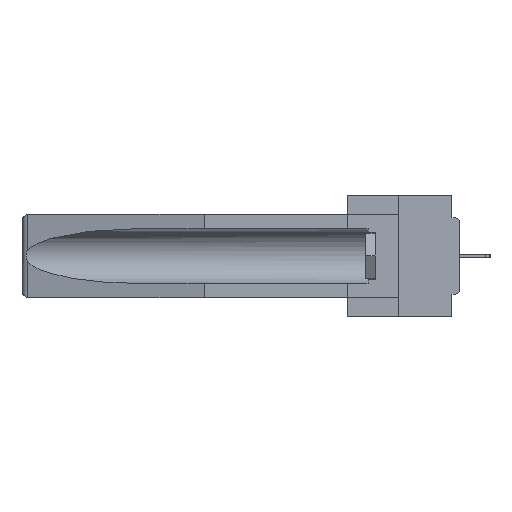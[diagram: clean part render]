
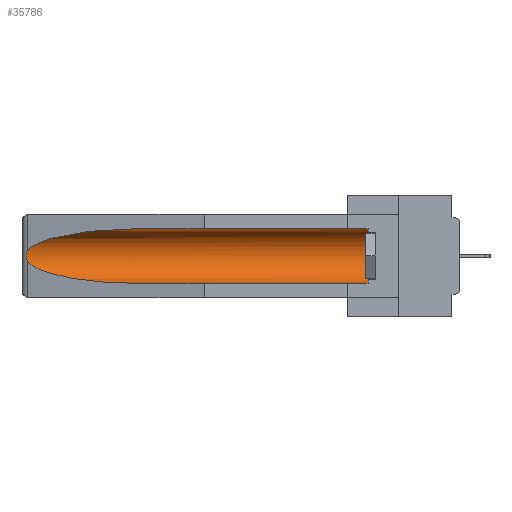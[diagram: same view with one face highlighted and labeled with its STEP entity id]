
A CAD part, left-side view. The second image highlights one B-rep face of the part: STEP entity #35786.
In plain terms, the highlighted cylindrical face has radius 2.857 mm (diameter 5.715 mm), a partial arc.
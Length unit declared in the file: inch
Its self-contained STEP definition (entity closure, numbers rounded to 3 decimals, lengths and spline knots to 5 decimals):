
#1238 = ORIENTED_EDGE ( 'NONE', *, *, #17198, .T. ) ;
#1365 = CARTESIAN_POINT ( 'NONE',  ( 0.2675, 1.53308, -0.16763 ) ) ;
#1535 = CYLINDRICAL_SURFACE ( 'NONE', #30972, 0.1125 ) ;
#1634 = VERTEX_POINT ( 'NONE', #39912 ) ;
#2962 = VERTEX_POINT ( 'NONE', #6089 ) ;
#3725 = CARTESIAN_POINT ( 'NONE',  ( 0.25451, 1.48313, -0.09465 ) ) ;
#5083 = CARTESIAN_POINT ( 'NONE',  ( 0.25451, 1.48313, -0.24835 ) ) ;
#6089 = CARTESIAN_POINT ( 'NONE',  ( 0.26537, 1.52718, -0.14972 ) ) ;
#6209 = ORIENTED_EDGE ( 'NONE', *, *, #26342, .T. ) ;
#6942 = CARTESIAN_POINT ( 'NONE',  ( 0.26654, 1.53092, -0.15636 ) ) ;
#7159 = EDGE_CURVE ( 'NONE', #2962, #30485, #22991, .T. ) ;
#7754 = CARTESIAN_POINT ( 'NONE',  ( 0.2673, 1.5327, -0.16383 ) ) ;
#8369 = CARTESIAN_POINT ( 'NONE',  ( 0.26537, 1.52718, -0.19328 ) ) ;
#9298 = DIRECTION ( 'NONE',  ( 0., 1., 0. ) ) ;
#13193 = CIRCLE ( 'NONE', #38894, 0.1125 ) ;
#13737 = CARTESIAN_POINT ( 'NONE',  ( 0.26537, 1.52718, -0.19328 ) ) ;
#13945 = CARTESIAN_POINT ( 'NONE',  ( 0.2673, 1.53269, -0.17917 ) ) ;
#15667 = CARTESIAN_POINT ( 'NONE',  ( 0.21114, 1.30732, -0.059 ) ) ;
#16207 = CARTESIAN_POINT ( 'NONE',  ( 0.26537, 1.52718, -0.19328 ) ) ;
#16802 = DIRECTION ( 'NONE',  ( 0., 0., 1. ) ) ;
#17198 = EDGE_CURVE ( 'NONE', #30485, #33576, #36864, .T. ) ;
#17990 = EDGE_LOOP ( 'NONE', ( #40339, #29797, #1238, #39306, #20578, #6209 ) ) ;
#18491 = CARTESIAN_POINT ( 'NONE',  ( 0.155, 0.126, -0.1715 ) ) ;
#19200 = CARTESIAN_POINT ( 'NONE',  ( 0.155, -0.30754, -0.284 ) ) ;
#20293 = DIRECTION ( 'NONE',  ( 0., 1., 0. ) ) ;
#20578 = ORIENTED_EDGE ( 'NONE', *, *, #23959, .T. ) ;
#20590 = CARTESIAN_POINT ( 'NONE',  ( 0.155, 1.07973, -0.284 ) ) ;
#20942 = CARTESIAN_POINT ( 'NONE',  ( 0.21114, 1.30732, -0.284 ) ) ;
#21858 = CARTESIAN_POINT ( 'NONE',  ( 0.155, 1.07973, -0.059 ) ) ;
#22188 = DIRECTION ( 'NONE',  ( 0., -1., 0. ) ) ;
#22264 = LINE ( 'NONE', #19200, #25817 ) ;
#22798 = CARTESIAN_POINT ( 'NONE',  ( 0.26597, 1.5296, -0.19026 ) ) ;
#22991 = B_SPLINE_CURVE_WITH_KNOTS ( 'NONE', 3,
 ( #29614, #35995, #6942, #7754, #1365, #29401, #13945, #38486, #22798, #13737 ),
 .UNSPECIFIED., .F., .F.,
 ( 4, 2, 2, 2, 4 ),
 ( 0., 0.00029, 0.00058, 0.00087, 0.00117 ),
 .UNSPECIFIED. ) ;
#23959 = EDGE_CURVE ( 'NONE', #37185, #1634, #13193, .T. ) ;
#24112 = VERTEX_POINT ( 'NONE', #38283 ) ;
#25548 = EDGE_CURVE ( 'NONE', #24112, #2962, #36615, .T. ) ;
#25605 = CARTESIAN_POINT ( 'NONE',  ( 0.155, -0.30754, -0.059 ) ) ;
#25817 = VECTOR ( 'NONE', #9298, 39.37008 ) ;
#26342 = EDGE_CURVE ( 'NONE', #1634, #24112, #28913, .T. ) ;
#27338 = CARTESIAN_POINT ( 'NONE',  ( 0.155, 1.07973, -0.284 ) ) ;
#28424 = VECTOR ( 'NONE', #35107, 39.37008 ) ;
#28715 = CARTESIAN_POINT ( 'NONE',  ( 0.155, 0.126, -0.284 ) ) ;
#28913 = LINE ( 'NONE', #25605, #28424 ) ;
#29401 = CARTESIAN_POINT ( 'NONE',  ( 0.2675, 1.53308, -0.17534 ) ) ;
#29614 = CARTESIAN_POINT ( 'NONE',  ( 0.26537, 1.52718, -0.14972 ) ) ;
#29774 = FACE_OUTER_BOUND ( 'NONE', #17990, .T. ) ;
#29797 = ORIENTED_EDGE ( 'NONE', *, *, #7159, .T. ) ;
#30485 = VERTEX_POINT ( 'NONE', #16207 ) ;
#30866 = DIRECTION ( 'NONE',  ( 0., 0., 1. ) ) ;
#30972 = AXIS2_PLACEMENT_3D ( 'NONE', #32465, #20293, #16802 ) ;
#31139 = CARTESIAN_POINT ( 'NONE',  ( 0.26537, 1.52718, -0.14972 ) ) ;
#32465 = CARTESIAN_POINT ( 'NONE',  ( 0.155, -0.30754, -0.1715 ) ) ;
#33576 = VERTEX_POINT ( 'NONE', #20590 ) ;
#35107 = DIRECTION ( 'NONE',  ( 0., 1., 0. ) ) ;
#35786 = ADVANCED_FACE ( 'NONE', ( #29774 ), #1535, .F. ) ;
#35995 = CARTESIAN_POINT ( 'NONE',  ( 0.26597, 1.52961, -0.15275 ) ) ;
#36615 =( BOUNDED_CURVE ( )  B_SPLINE_CURVE ( 3, ( #21858, #15667, #3725, #31139 ),
 .UNSPECIFIED., .F., .F. ) 
 B_SPLINE_CURVE_WITH_KNOTS ( ( 4, 4 ),
 ( 4.71239, 6.08839 ),
 .UNSPECIFIED. ) 
 CURVE ( )  GEOMETRIC_REPRESENTATION_ITEM ( )  RATIONAL_B_SPLINE_CURVE ( ( 1., 0.848, 0.848, 1. ) ) 
 REPRESENTATION_ITEM ( '' )  );
#36864 =( BOUNDED_CURVE ( )  B_SPLINE_CURVE ( 3, ( #8369, #5083, #20942, #27338 ),
 .UNSPECIFIED., .F., .F. ) 
 B_SPLINE_CURVE_WITH_KNOTS ( ( 4, 4 ),
 ( 0.1948, 1.5708 ),
 .UNSPECIFIED. ) 
 CURVE ( )  GEOMETRIC_REPRESENTATION_ITEM ( )  RATIONAL_B_SPLINE_CURVE ( ( 1., 0.848, 0.848, 1. ) ) 
 REPRESENTATION_ITEM ( '' )  );
#37185 = VERTEX_POINT ( 'NONE', #28715 ) ;
#37605 = EDGE_CURVE ( 'NONE', #37185, #33576, #22264, .T. ) ;
#38283 = CARTESIAN_POINT ( 'NONE',  ( 0.155, 1.07973, -0.059 ) ) ;
#38486 = CARTESIAN_POINT ( 'NONE',  ( 0.26655, 1.53094, -0.18657 ) ) ;
#38894 = AXIS2_PLACEMENT_3D ( 'NONE', #18491, #22188, #30866 ) ;
#39306 = ORIENTED_EDGE ( 'NONE', *, *, #37605, .F. ) ;
#39912 = CARTESIAN_POINT ( 'NONE',  ( 0.155, 0.126, -0.059 ) ) ;
#40339 = ORIENTED_EDGE ( 'NONE', *, *, #25548, .T. ) ;
